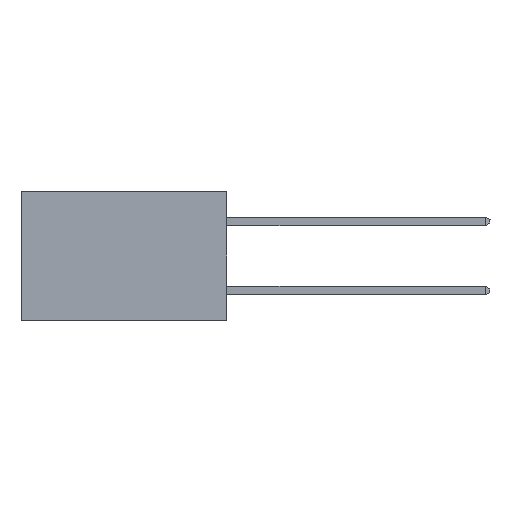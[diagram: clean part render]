
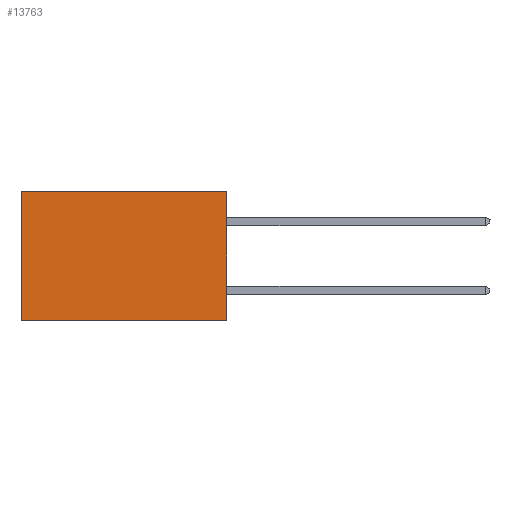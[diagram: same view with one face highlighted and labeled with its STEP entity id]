
A CAD part, left-side view. The second image highlights one B-rep face of the part: STEP entity #13763.
In plain terms, the highlighted planar face has unit normal (-1, 0, 0).
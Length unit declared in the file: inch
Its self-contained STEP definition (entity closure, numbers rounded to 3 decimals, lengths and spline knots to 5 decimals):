
#2867 = DIRECTION ( 'NONE',  ( 0., 1., 0. ) ) ;
#2919 = CARTESIAN_POINT ( 'NONE',  ( 0.277, 0.59, -0.37 ) ) ;
#3269 = DIRECTION ( 'NONE',  ( 0., 1., 0. ) ) ;
#3331 = CARTESIAN_POINT ( 'NONE',  ( 0.277, 0., -0.37 ) ) ;
#4147 = CARTESIAN_POINT ( 'NONE',  ( 0.277, 0.59, -0.37 ) ) ;
#4150 = VECTOR ( 'NONE', #2867, 39.37008 ) ;
#4178 = LINE ( 'NONE', #2919, #15611 ) ;
#4723 = PLANE ( 'NONE',  #6995 ) ;
#4787 = DIRECTION ( 'NONE',  ( 1., 0., 0. ) ) ;
#6206 = ORIENTED_EDGE ( 'NONE', *, *, #8193, .F. ) ;
#6867 = CARTESIAN_POINT ( 'NONE',  ( 0.277, 0., -0.37 ) ) ;
#6951 = VECTOR ( 'NONE', #3269, 39.37008 ) ;
#6995 = AXIS2_PLACEMENT_3D ( 'NONE', #10708, #4787, #15230 ) ;
#7112 = VECTOR ( 'NONE', #8312, 39.37008 ) ;
#7305 = EDGE_CURVE ( 'NONE', #8225, #9415, #4178, .T. ) ;
#7917 = CARTESIAN_POINT ( 'NONE',  ( 0.277, 0.59, 0. ) ) ;
#8088 = ORIENTED_EDGE ( 'NONE', *, *, #16896, .F. ) ;
#8193 = EDGE_CURVE ( 'NONE', #16976, #9415, #14875, .T. ) ;
#8225 = VERTEX_POINT ( 'NONE', #7917 ) ;
#8312 = DIRECTION ( 'NONE',  ( 0., 0., -1. ) ) ;
#8896 = DIRECTION ( 'NONE',  ( 0., 0., -1. ) ) ;
#9415 = VERTEX_POINT ( 'NONE', #4147 ) ;
#10292 = CARTESIAN_POINT ( 'NONE',  ( 0.277, 0., 0. ) ) ;
#10708 = CARTESIAN_POINT ( 'NONE',  ( 0.277, 0., -0.37 ) ) ;
#10853 = EDGE_LOOP ( 'NONE', ( #17178, #6206, #8088, #16504 ) ) ;
#11339 = CARTESIAN_POINT ( 'NONE',  ( 0.277, 0., 0. ) ) ;
#12044 = LINE ( 'NONE', #10292, #4150 ) ;
#13763 = ADVANCED_FACE ( 'NONE', ( #17027 ), #4723, .F. ) ;
#14875 = LINE ( 'NONE', #3331, #6951 ) ;
#14983 = EDGE_CURVE ( 'NONE', #18797, #8225, #12044, .T. ) ;
#15230 = DIRECTION ( 'NONE',  ( 0., 0., -1. ) ) ;
#15611 = VECTOR ( 'NONE', #8896, 39.37008 ) ;
#16013 = CARTESIAN_POINT ( 'NONE',  ( 0.277, 0., -0.37 ) ) ;
#16504 = ORIENTED_EDGE ( 'NONE', *, *, #14983, .T. ) ;
#16896 = EDGE_CURVE ( 'NONE', #18797, #16976, #18528, .T. ) ;
#16976 = VERTEX_POINT ( 'NONE', #16013 ) ;
#17027 = FACE_OUTER_BOUND ( 'NONE', #10853, .T. ) ;
#17178 = ORIENTED_EDGE ( 'NONE', *, *, #7305, .T. ) ;
#18528 = LINE ( 'NONE', #6867, #7112 ) ;
#18797 = VERTEX_POINT ( 'NONE', #11339 ) ;
